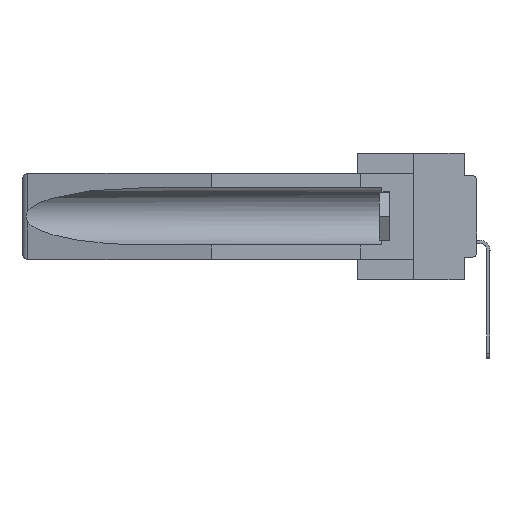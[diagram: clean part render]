
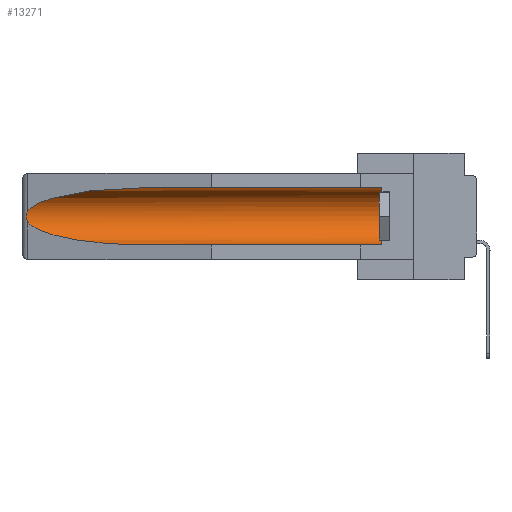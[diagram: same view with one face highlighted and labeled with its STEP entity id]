
A CAD part, left-side view. The second image highlights one B-rep face of the part: STEP entity #13271.
In plain terms, the highlighted cylindrical face has radius 2.857 mm (diameter 5.715 mm), a partial arc.
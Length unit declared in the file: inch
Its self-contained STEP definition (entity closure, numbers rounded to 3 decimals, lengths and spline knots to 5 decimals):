
#889 = CARTESIAN_POINT ( 'NONE',  ( 0.2673, 1.5327, -0.16383 ) ) ;
#1939 =( BOUNDED_CURVE ( )  B_SPLINE_CURVE ( 3, ( #17803, #6347, #26979, #20209 ),
 .UNSPECIFIED., .F., .T. ) 
 B_SPLINE_CURVE_WITH_KNOTS ( ( 4, 4 ),
 ( 4.71239, 6.08839 ),
 .UNSPECIFIED. ) 
 CURVE ( )  GEOMETRIC_REPRESENTATION_ITEM ( )  RATIONAL_B_SPLINE_CURVE ( ( 1., 0.848, 0.848, 1. ) ) 
 REPRESENTATION_ITEM ( '' )  );
#2016 = CARTESIAN_POINT ( 'NONE',  ( 0.155, 1.07973, -0.284 ) ) ;
#3354 = DIRECTION ( 'NONE',  ( 0., -1., 0. ) ) ;
#3611 = CARTESIAN_POINT ( 'NONE',  ( 0.21114, 1.30732, -0.284 ) ) ;
#3962 = EDGE_CURVE ( 'NONE', #26042, #15669, #15239, .T. ) ;
#5415 = VERTEX_POINT ( 'NONE', #14593 ) ;
#5707 = CARTESIAN_POINT ( 'NONE',  ( 0.26654, 1.53092, -0.15636 ) ) ;
#5994 = CARTESIAN_POINT ( 'NONE',  ( 0.26597, 1.52961, -0.15275 ) ) ;
#6149 = ORIENTED_EDGE ( 'NONE', *, *, #12695, .T. ) ;
#6347 = CARTESIAN_POINT ( 'NONE',  ( 0.21114, 1.30732, -0.059 ) ) ;
#6468 = EDGE_CURVE ( 'NONE', #26334, #26042, #24801, .T. ) ;
#7680 = VECTOR ( 'NONE', #27736, 39.37008 ) ;
#7688 = LINE ( 'NONE', #16889, #7680 ) ;
#8018 = DIRECTION ( 'NONE',  ( 0., 0., 1. ) ) ;
#8115 = CARTESIAN_POINT ( 'NONE',  ( 0.26597, 1.5296, -0.19026 ) ) ;
#8121 = CARTESIAN_POINT ( 'NONE',  ( 0.26537, 1.52718, -0.14972 ) ) ;
#9255 = VERTEX_POINT ( 'NONE', #21196 ) ;
#10394 = CARTESIAN_POINT ( 'NONE',  ( 0.26537, 1.52718, -0.14972 ) ) ;
#10755 = DIRECTION ( 'NONE',  ( 0., 1., 0. ) ) ;
#11293 = CARTESIAN_POINT ( 'NONE',  ( 0.155, 1.07973, -0.284 ) ) ;
#12695 = EDGE_CURVE ( 'NONE', #9255, #23879, #22026, .T. ) ;
#13271 = ADVANCED_FACE ( 'NONE', ( #29521 ), #29076, .F. ) ;
#13656 = AXIS2_PLACEMENT_3D ( 'NONE', #26392, #3354, #8018 ) ;
#14593 = CARTESIAN_POINT ( 'NONE',  ( 0.155, 0.126, -0.284 ) ) ;
#14760 = CARTESIAN_POINT ( 'NONE',  ( 0.26655, 1.53094, -0.18657 ) ) ;
#15064 = CARTESIAN_POINT ( 'NONE',  ( 0.26537, 1.52718, -0.19328 ) ) ;
#15239 =( BOUNDED_CURVE ( )  B_SPLINE_CURVE ( 3, ( #15064, #24234, #3611, #11293 ),
 .UNSPECIFIED., .F., .T. ) 
 B_SPLINE_CURVE_WITH_KNOTS ( ( 4, 4 ),
 ( 0.1948, 1.5708 ),
 .UNSPECIFIED. ) 
 CURVE ( )  GEOMETRIC_REPRESENTATION_ITEM ( )  RATIONAL_B_SPLINE_CURVE ( ( 1., 0.848, 0.848, 1. ) ) 
 REPRESENTATION_ITEM ( '' )  );
#15669 = VERTEX_POINT ( 'NONE', #2016 ) ;
#15911 = EDGE_CURVE ( 'NONE', #23879, #26334, #1939, .T. ) ;
#16889 = CARTESIAN_POINT ( 'NONE',  ( 0.155, -0.30754, -0.284 ) ) ;
#17462 = AXIS2_PLACEMENT_3D ( 'NONE', #29376, #29678, #22432 ) ;
#17803 = CARTESIAN_POINT ( 'NONE',  ( 0.155, 1.07973, -0.059 ) ) ;
#19129 = CARTESIAN_POINT ( 'NONE',  ( 0.2673, 1.53269, -0.17917 ) ) ;
#19565 = CARTESIAN_POINT ( 'NONE',  ( 0.2675, 1.53308, -0.16763 ) ) ;
#20209 = CARTESIAN_POINT ( 'NONE',  ( 0.26537, 1.52718, -0.14972 ) ) ;
#20381 = CIRCLE ( 'NONE', #13656, 0.1125 ) ;
#20983 = ORIENTED_EDGE ( 'NONE', *, *, #6468, .T. ) ;
#21036 = ORIENTED_EDGE ( 'NONE', *, *, #3962, .T. ) ;
#21196 = CARTESIAN_POINT ( 'NONE',  ( 0.155, 0.126, -0.059 ) ) ;
#21325 = EDGE_LOOP ( 'NONE', ( #25326, #20983, #21036, #24541, #26479, #6149 ) ) ;
#22026 = LINE ( 'NONE', #29115, #29554 ) ;
#22432 = DIRECTION ( 'NONE',  ( 0., 0., 1. ) ) ;
#23035 = CARTESIAN_POINT ( 'NONE',  ( 0.26537, 1.52718, -0.19328 ) ) ;
#23741 = EDGE_CURVE ( 'NONE', #5415, #15669, #7688, .T. ) ;
#23879 = VERTEX_POINT ( 'NONE', #26210 ) ;
#24234 = CARTESIAN_POINT ( 'NONE',  ( 0.25451, 1.48313, -0.24835 ) ) ;
#24541 = ORIENTED_EDGE ( 'NONE', *, *, #23741, .F. ) ;
#24801 = B_SPLINE_CURVE_WITH_KNOTS ( 'NONE', 3,
 ( #10394, #5994, #5707, #889, #19565, #28739, #19129, #14760, #8115, #26193 ),
 .UNSPECIFIED., .F., .F.,
 ( 4, 2, 2, 2, 4 ),
 ( 0., 0.00029, 0.00058, 0.00087, 0.00117 ),
 .UNSPECIFIED. ) ;
#25326 = ORIENTED_EDGE ( 'NONE', *, *, #15911, .T. ) ;
#26042 = VERTEX_POINT ( 'NONE', #23035 ) ;
#26193 = CARTESIAN_POINT ( 'NONE',  ( 0.26537, 1.52718, -0.19328 ) ) ;
#26210 = CARTESIAN_POINT ( 'NONE',  ( 0.155, 1.07973, -0.059 ) ) ;
#26334 = VERTEX_POINT ( 'NONE', #8121 ) ;
#26392 = CARTESIAN_POINT ( 'NONE',  ( 0.155, 0.126, -0.1715 ) ) ;
#26479 = ORIENTED_EDGE ( 'NONE', *, *, #28873, .T. ) ;
#26979 = CARTESIAN_POINT ( 'NONE',  ( 0.25451, 1.48313, -0.09465 ) ) ;
#27736 = DIRECTION ( 'NONE',  ( 0., 1., 0. ) ) ;
#28739 = CARTESIAN_POINT ( 'NONE',  ( 0.2675, 1.53308, -0.17534 ) ) ;
#28873 = EDGE_CURVE ( 'NONE', #5415, #9255, #20381, .T. ) ;
#29076 = CYLINDRICAL_SURFACE ( 'NONE', #17462, 0.1125 ) ;
#29115 = CARTESIAN_POINT ( 'NONE',  ( 0.155, -0.30754, -0.059 ) ) ;
#29376 = CARTESIAN_POINT ( 'NONE',  ( 0.155, -0.30754, -0.1715 ) ) ;
#29521 = FACE_OUTER_BOUND ( 'NONE', #21325, .T. ) ;
#29554 = VECTOR ( 'NONE', #10755, 39.37008 ) ;
#29678 = DIRECTION ( 'NONE',  ( 0., 1., 0. ) ) ;
